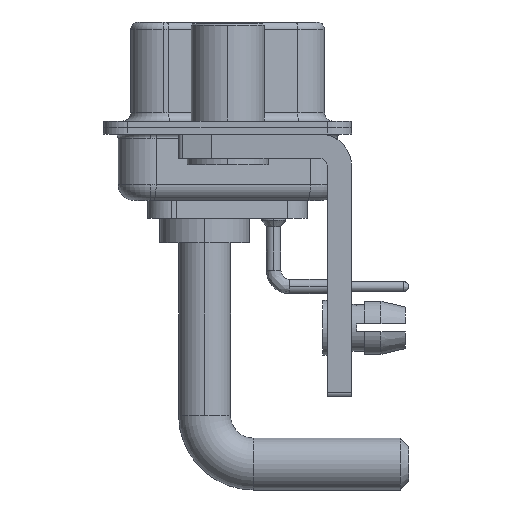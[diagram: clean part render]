
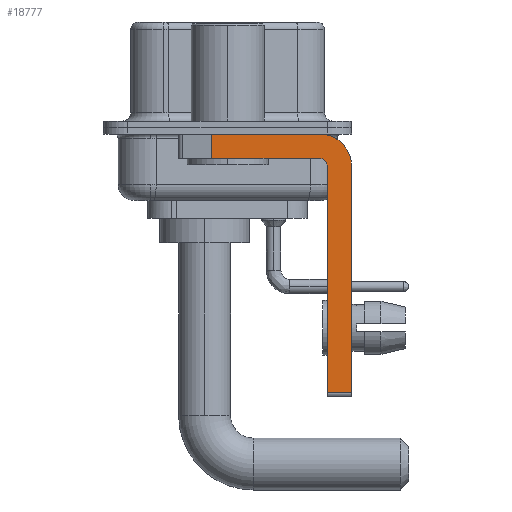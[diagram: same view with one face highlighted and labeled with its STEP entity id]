
A CAD part, left-side view. The second image highlights one B-rep face of the part: STEP entity #18777.
In plain terms, the highlighted planar face has unit normal (-1, 0, 0).
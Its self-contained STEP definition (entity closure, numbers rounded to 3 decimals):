
#200 = DIRECTION ( 'NONE',  ( 0., 0., 1. ) ) ;
#334 = DIRECTION ( 'NONE',  ( 0., -1., 0. ) ) ;
#350 = VECTOR ( 'NONE', #11907, 1000. ) ;
#1247 = ORIENTED_EDGE ( 'NONE', *, *, #18483, .F. ) ;
#1770 = DIRECTION ( 'NONE',  ( 1., 0., 0. ) ) ;
#2226 = EDGE_CURVE ( 'NONE', #27653, #5441, #12363, .T. ) ;
#2388 = EDGE_CURVE ( 'NONE', #3656, #16993, #15433, .T. ) ;
#3471 = CARTESIAN_POINT ( 'NONE',  ( -2.9, -5.65, -1.9 ) ) ;
#3656 = VERTEX_POINT ( 'NONE', #16300 ) ;
#4145 = EDGE_CURVE ( 'NONE', #18643, #5441, #16681, .T. ) ;
#4324 = VECTOR ( 'NONE', #13240, 1000. ) ;
#4609 = LINE ( 'NONE', #11441, #23544 ) ;
#5441 = VERTEX_POINT ( 'NONE', #12189 ) ;
#6726 = LINE ( 'NONE', #15234, #26329 ) ;
#7532 = ORIENTED_EDGE ( 'NONE', *, *, #2226, .T. ) ;
#7782 = ORIENTED_EDGE ( 'NONE', *, *, #19028, .F. ) ;
#7984 = VERTEX_POINT ( 'NONE', #11495 ) ;
#8028 = PLANE ( 'NONE',  #24976 ) ;
#9116 = ORIENTED_EDGE ( 'NONE', *, *, #4145, .F. ) ;
#10038 = CARTESIAN_POINT ( 'NONE',  ( -2.9, -5.65, -1.9 ) ) ;
#10432 = FACE_OUTER_BOUND ( 'NONE', #20762, .T. ) ;
#11441 = CARTESIAN_POINT ( 'NONE',  ( -2.9, -7.65, -2.4 ) ) ;
#11495 = CARTESIAN_POINT ( 'NONE',  ( -2.9, -7.65, -2.4 ) ) ;
#11907 = DIRECTION ( 'NONE',  ( 0., 1., 0. ) ) ;
#12072 = EDGE_CURVE ( 'NONE', #3656, #12993, #24144, .T. ) ;
#12189 = CARTESIAN_POINT ( 'NONE',  ( -2.9, 0.978, -1.9 ) ) ;
#12363 = LINE ( 'NONE', #19411, #25994 ) ;
#12744 = EDGE_CURVE ( 'NONE', #12993, #18643, #24279, .T. ) ;
#12946 = VECTOR ( 'NONE', #13323, 1000. ) ;
#12993 = VERTEX_POINT ( 'NONE', #17903 ) ;
#13240 = DIRECTION ( 'NONE',  ( 0., 0., 1. ) ) ;
#13323 = DIRECTION ( 'NONE',  ( 0., -1., 0. ) ) ;
#13695 = DIRECTION ( 'NONE',  ( 0., 0., -1. ) ) ;
#13900 = EDGE_CURVE ( 'NONE', #21563, #7984, #14397, .T. ) ;
#14397 = CIRCLE ( 'NONE', #27499, 2. ) ;
#15234 = CARTESIAN_POINT ( 'NONE',  ( -2.9, 3., -0.4 ) ) ;
#15433 = LINE ( 'NONE', #17685, #12946 ) ;
#16300 = CARTESIAN_POINT ( 'NONE',  ( -2.9, -6.15, -16.35 ) ) ;
#16681 = LINE ( 'NONE', #10038, #350 ) ;
#16993 = VERTEX_POINT ( 'NONE', #20232 ) ;
#17028 = AXIS2_PLACEMENT_3D ( 'NONE', #17209, #22025, #200 ) ;
#17209 = CARTESIAN_POINT ( 'NONE',  ( -2.9, -5.65, -2.4 ) ) ;
#17227 = ORIENTED_EDGE ( 'NONE', *, *, #2388, .T. ) ;
#17685 = CARTESIAN_POINT ( 'NONE',  ( -2.9, -5.65, -16.35 ) ) ;
#17903 = CARTESIAN_POINT ( 'NONE',  ( -2.9, -6.15, -2.4 ) ) ;
#17958 = CARTESIAN_POINT ( 'NONE',  ( -2.9, -5.65, -0.4 ) ) ;
#18483 = EDGE_CURVE ( 'NONE', #7984, #16993, #4609, .T. ) ;
#18643 = VERTEX_POINT ( 'NONE', #3471 ) ;
#18777 = ADVANCED_FACE ( 'NONE', ( #10432 ), #8028, .F. ) ;
#19028 = EDGE_CURVE ( 'NONE', #27653, #21563, #6726, .T. ) ;
#19125 = DIRECTION ( 'NONE',  ( 0., 0., -1. ) ) ;
#19206 = DIRECTION ( 'NONE',  ( 0., 0., -1. ) ) ;
#19411 = CARTESIAN_POINT ( 'NONE',  ( -2.9, 0.978, -1.9 ) ) ;
#20104 = ORIENTED_EDGE ( 'NONE', *, *, #12072, .F. ) ;
#20232 = CARTESIAN_POINT ( 'NONE',  ( -2.9, -7.65, -16.35 ) ) ;
#20249 = ORIENTED_EDGE ( 'NONE', *, *, #12744, .F. ) ;
#20762 = EDGE_LOOP ( 'NONE', ( #7782, #7532, #9116, #20249, #20104, #17227, #1247, #26579 ) ) ;
#21471 = CARTESIAN_POINT ( 'NONE',  ( -2.9, -5.65, -2.4 ) ) ;
#21563 = VERTEX_POINT ( 'NONE', #17958 ) ;
#22025 = DIRECTION ( 'NONE',  ( -1., 0., 0. ) ) ;
#22706 = CARTESIAN_POINT ( 'NONE',  ( -2.9, 0.978, -0.4 ) ) ;
#23455 = CARTESIAN_POINT ( 'NONE',  ( -2.9, -5.65, -2.4 ) ) ;
#23544 = VECTOR ( 'NONE', #13695, 1000. ) ;
#24014 = CARTESIAN_POINT ( 'NONE',  ( -2.9, -6.15, -16.6 ) ) ;
#24144 = LINE ( 'NONE', #24014, #4324 ) ;
#24279 = CIRCLE ( 'NONE', #17028, 0.5 ) ;
#24976 = AXIS2_PLACEMENT_3D ( 'NONE', #23455, #27570, #25436 ) ;
#25436 = DIRECTION ( 'NONE',  ( 0., 0., -1. ) ) ;
#25994 = VECTOR ( 'NONE', #19125, 1000. ) ;
#26329 = VECTOR ( 'NONE', #334, 1000. ) ;
#26579 = ORIENTED_EDGE ( 'NONE', *, *, #13900, .F. ) ;
#27499 = AXIS2_PLACEMENT_3D ( 'NONE', #21471, #1770, #19206 ) ;
#27570 = DIRECTION ( 'NONE',  ( 1., 0., 0. ) ) ;
#27653 = VERTEX_POINT ( 'NONE', #22706 ) ;
